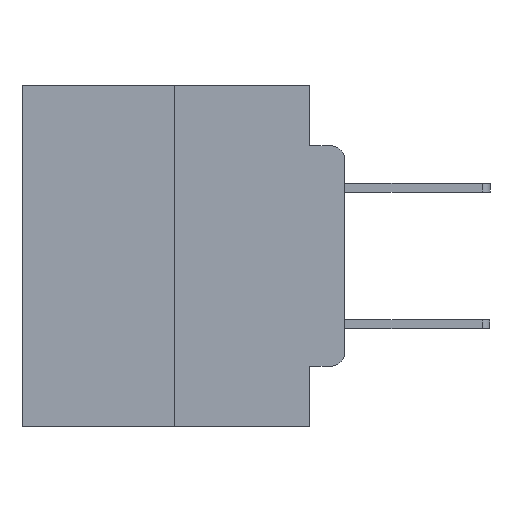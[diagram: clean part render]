
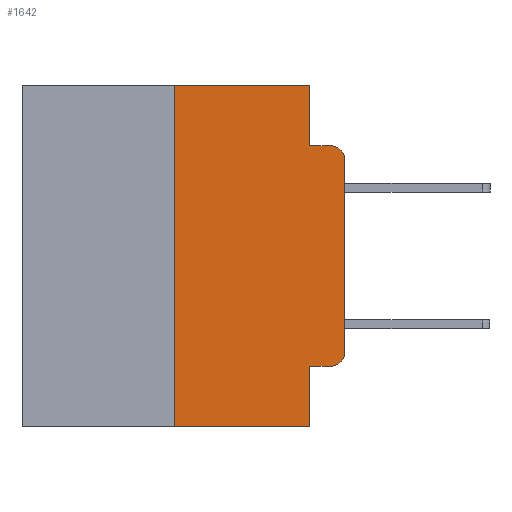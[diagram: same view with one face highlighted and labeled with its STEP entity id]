
A CAD part, left-side view. The second image highlights one B-rep face of the part: STEP entity #1642.
In plain terms, the highlighted planar face has unit normal (-1, 0, 0).
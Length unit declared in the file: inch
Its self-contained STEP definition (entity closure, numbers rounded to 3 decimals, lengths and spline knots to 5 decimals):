
#496 = VECTOR ( 'NONE', #21173, 39.37008 ) ;
#579 = VERTEX_POINT ( 'NONE', #14480 ) ;
#888 = VERTEX_POINT ( 'NONE', #23103 ) ;
#985 = ORIENTED_EDGE ( 'NONE', *, *, #16563, .T. ) ;
#1000 = CARTESIAN_POINT ( 'NONE',  ( 0., 0.051, -0.5 ) ) ;
#1309 = EDGE_CURVE ( 'NONE', #17049, #5979, #24650, .T. ) ;
#1314 = LINE ( 'NONE', #21437, #7573 ) ;
#1642 = ADVANCED_FACE ( 'NONE', ( #7405 ), #15698, .F. ) ;
#1653 = DIRECTION ( 'NONE',  ( 0., 0., -1. ) ) ;
#2379 = DIRECTION ( 'NONE',  ( 1., 0., 0. ) ) ;
#2765 = CARTESIAN_POINT ( 'NONE',  ( 0., 0.02, -0.3915 ) ) ;
#3609 = LINE ( 'NONE', #5669, #13857 ) ;
#3647 = AXIS2_PLACEMENT_3D ( 'NONE', #24784, #2379, #24416 ) ;
#3819 = VERTEX_POINT ( 'NONE', #19735 ) ;
#4109 = VECTOR ( 'NONE', #25565, 39.37008 ) ;
#4186 = CIRCLE ( 'NONE', #17493, 0.02 ) ;
#4757 = CARTESIAN_POINT ( 'NONE',  ( 0., 0.473, -0.5 ) ) ;
#4894 = DIRECTION ( 'NONE',  ( 0., 0., -1. ) ) ;
#5274 = LINE ( 'NONE', #10878, #15525 ) ;
#5669 = CARTESIAN_POINT ( 'NONE',  ( 0., 0.473, 0. ) ) ;
#5979 = VERTEX_POINT ( 'NONE', #15869 ) ;
#6281 = ORIENTED_EDGE ( 'NONE', *, *, #22683, .F. ) ;
#6458 = EDGE_LOOP ( 'NONE', ( #7270, #985, #9198, #6926, #6281, #13608, #16866, #12326, #12972, #15890 ) ) ;
#6511 = CARTESIAN_POINT ( 'NONE',  ( 0., 0., -0.1085 ) ) ;
#6792 = LINE ( 'NONE', #4757, #496 ) ;
#6926 = ORIENTED_EDGE ( 'NONE', *, *, #1309, .F. ) ;
#7106 = DIRECTION ( 'NONE',  ( 0., -1., 0. ) ) ;
#7270 = ORIENTED_EDGE ( 'NONE', *, *, #17938, .T. ) ;
#7400 = DIRECTION ( 'NONE',  ( 0., -1., 0. ) ) ;
#7405 = FACE_OUTER_BOUND ( 'NONE', #6458, .T. ) ;
#7573 = VECTOR ( 'NONE', #7106, 39.37008 ) ;
#7754 = DIRECTION ( 'NONE',  ( 0., -1., 0. ) ) ;
#7992 = CARTESIAN_POINT ( 'NONE',  ( 0., 0.051, 0. ) ) ;
#8368 = VECTOR ( 'NONE', #9841, 39.37008 ) ;
#8944 = LINE ( 'NONE', #11314, #4109 ) ;
#9198 = ORIENTED_EDGE ( 'NONE', *, *, #9685, .F. ) ;
#9447 = CARTESIAN_POINT ( 'NONE',  ( 0., 0.051, -0.0885 ) ) ;
#9685 = EDGE_CURVE ( 'NONE', #5979, #888, #26438, .T. ) ;
#9841 = DIRECTION ( 'NONE',  ( 0., 0., -1. ) ) ;
#10041 = CARTESIAN_POINT ( 'NONE',  ( 0., 0.051, 0. ) ) ;
#10233 = VECTOR ( 'NONE', #7400, 39.37008 ) ;
#10878 = CARTESIAN_POINT ( 'NONE',  ( 0., 0.25, 0. ) ) ;
#11002 = CARTESIAN_POINT ( 'NONE',  ( 0., 0.02, -0.1085 ) ) ;
#11155 = VERTEX_POINT ( 'NONE', #1000 ) ;
#11314 = CARTESIAN_POINT ( 'NONE',  ( 0., 0., 0. ) ) ;
#11565 = EDGE_CURVE ( 'NONE', #20804, #3819, #13676, .T. ) ;
#11813 = CARTESIAN_POINT ( 'NONE',  ( 0., 0.25, -0.5 ) ) ;
#11904 = AXIS2_PLACEMENT_3D ( 'NONE', #2765, #17198, #4894 ) ;
#12326 = ORIENTED_EDGE ( 'NONE', *, *, #19824, .F. ) ;
#12912 = EDGE_CURVE ( 'NONE', #13211, #20804, #1314, .T. ) ;
#12914 = DIRECTION ( 'NONE',  ( 0., 0., 1. ) ) ;
#12972 = ORIENTED_EDGE ( 'NONE', *, *, #12912, .T. ) ;
#13034 = DIRECTION ( 'NONE',  ( 0., 0., -1. ) ) ;
#13211 = VERTEX_POINT ( 'NONE', #22398 ) ;
#13608 = ORIENTED_EDGE ( 'NONE', *, *, #21191, .F. ) ;
#13676 = CIRCLE ( 'NONE', #11904, 0.02 ) ;
#13857 = VECTOR ( 'NONE', #7754, 39.37008 ) ;
#14480 = CARTESIAN_POINT ( 'NONE',  ( 0., 0.25, 0. ) ) ;
#15094 = VERTEX_POINT ( 'NONE', #6511 ) ;
#15525 = VECTOR ( 'NONE', #12914, 39.37008 ) ;
#15598 = LINE ( 'NONE', #16106, #21061 ) ;
#15698 = PLANE ( 'NONE',  #3647 ) ;
#15869 = CARTESIAN_POINT ( 'NONE',  ( 0., 0.051, -0.0885 ) ) ;
#15885 = EDGE_CURVE ( 'NONE', #24493, #11155, #6792, .T. ) ;
#15890 = ORIENTED_EDGE ( 'NONE', *, *, #11565, .T. ) ;
#16106 = CARTESIAN_POINT ( 'NONE',  ( 0., 0.051, 0. ) ) ;
#16563 = EDGE_CURVE ( 'NONE', #15094, #888, #4186, .T. ) ;
#16866 = ORIENTED_EDGE ( 'NONE', *, *, #15885, .T. ) ;
#17049 = VERTEX_POINT ( 'NONE', #7992 ) ;
#17198 = DIRECTION ( 'NONE',  ( -1., 0., 0. ) ) ;
#17493 = AXIS2_PLACEMENT_3D ( 'NONE', #11002, #25250, #13034 ) ;
#17938 = EDGE_CURVE ( 'NONE', #3819, #15094, #8944, .T. ) ;
#19735 = CARTESIAN_POINT ( 'NONE',  ( 0., 0., -0.3915 ) ) ;
#19824 = EDGE_CURVE ( 'NONE', #13211, #11155, #15598, .T. ) ;
#20804 = VERTEX_POINT ( 'NONE', #21633 ) ;
#21061 = VECTOR ( 'NONE', #1653, 39.37008 ) ;
#21173 = DIRECTION ( 'NONE',  ( 0., -1., 0. ) ) ;
#21191 = EDGE_CURVE ( 'NONE', #24493, #579, #5274, .T. ) ;
#21437 = CARTESIAN_POINT ( 'NONE',  ( 0., 0.051, -0.4115 ) ) ;
#21633 = CARTESIAN_POINT ( 'NONE',  ( 0., 0.02, -0.4115 ) ) ;
#22398 = CARTESIAN_POINT ( 'NONE',  ( 0., 0.051, -0.4115 ) ) ;
#22683 = EDGE_CURVE ( 'NONE', #579, #17049, #3609, .T. ) ;
#23103 = CARTESIAN_POINT ( 'NONE',  ( 0., 0.02, -0.0885 ) ) ;
#24416 = DIRECTION ( 'NONE',  ( 0., 0., -1. ) ) ;
#24493 = VERTEX_POINT ( 'NONE', #11813 ) ;
#24650 = LINE ( 'NONE', #10041, #8368 ) ;
#24784 = CARTESIAN_POINT ( 'NONE',  ( 0., 0.473, 0. ) ) ;
#25250 = DIRECTION ( 'NONE',  ( -1., 0., 0. ) ) ;
#25565 = DIRECTION ( 'NONE',  ( 0., 0., 1. ) ) ;
#26438 = LINE ( 'NONE', #9447, #10233 ) ;
